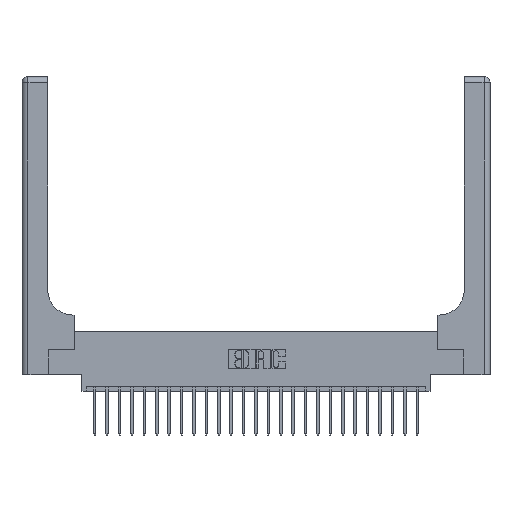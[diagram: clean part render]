
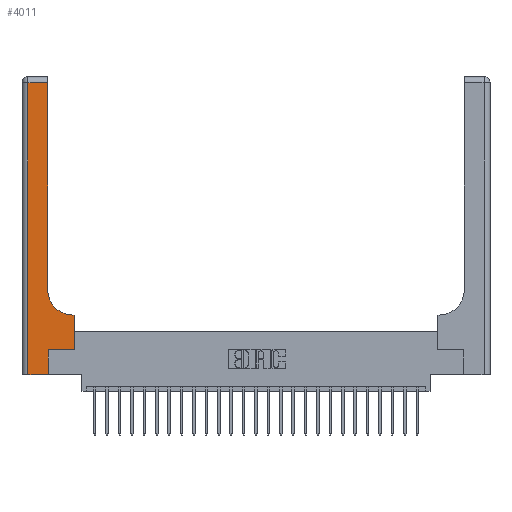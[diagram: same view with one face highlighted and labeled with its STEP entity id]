
A CAD part, top view. The second image highlights one B-rep face of the part: STEP entity #4011.
In plain terms, the highlighted planar face has unit normal (0, 0, 1).
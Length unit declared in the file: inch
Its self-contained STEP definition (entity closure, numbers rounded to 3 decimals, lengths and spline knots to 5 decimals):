
#607 = EDGE_CURVE ( 'NONE', #18740, #5531, #4757, .T. ) ;
#1061 = CARTESIAN_POINT ( 'NONE',  ( 0., 0., 0.37 ) ) ;
#1181 = DIRECTION ( 'NONE',  ( 0., 0., -1. ) ) ;
#1553 = VECTOR ( 'NONE', #13755, 39.37008 ) ;
#1917 = EDGE_CURVE ( 'NONE', #15763, #5478, #7448, .T. ) ;
#3031 = DIRECTION ( 'NONE',  ( 1., 0., 0. ) ) ;
#3609 = LINE ( 'NONE', #18284, #18433 ) ;
#4011 = ADVANCED_FACE ( 'NONE', ( #15959 ), #17779, .F. ) ;
#4052 = DIRECTION ( 'NONE',  ( -1., 0., 0. ) ) ;
#4178 = VERTEX_POINT ( 'NONE', #22391 ) ;
#4524 = EDGE_CURVE ( 'NONE', #15394, #18740, #11393, .T. ) ;
#4541 = CARTESIAN_POINT ( 'NONE',  ( 0.265, 0.25, 0.37 ) ) ;
#4726 = DIRECTION ( 'NONE',  ( 0., -1., 0. ) ) ;
#4745 = DIRECTION ( 'NONE',  ( 0., 1., 0. ) ) ;
#4757 = LINE ( 'NONE', #12441, #24632 ) ;
#4801 = LINE ( 'NONE', #1061, #14484 ) ;
#5115 = CARTESIAN_POINT ( 'NONE',  ( 0.26, 0.85, 0.37 ) ) ;
#5478 = VERTEX_POINT ( 'NONE', #5115 ) ;
#5531 = VERTEX_POINT ( 'NONE', #20825 ) ;
#5740 = VECTOR ( 'NONE', #16269, 39.37008 ) ;
#6201 = DIRECTION ( 'NONE',  ( 0., 0., -1. ) ) ;
#7081 = CARTESIAN_POINT ( 'NONE',  ( 0.528, 0.25, 0.37 ) ) ;
#7318 = LINE ( 'NONE', #11815, #1553 ) ;
#7344 = VERTEX_POINT ( 'NONE', #21788 ) ;
#7448 = CIRCLE ( 'NONE', #7459, 0.25 ) ;
#7459 = AXIS2_PLACEMENT_3D ( 'NONE', #12795, #1181, #14747 ) ;
#8339 = CARTESIAN_POINT ( 'NONE',  ( 0.26, 0.6, 0.37 ) ) ;
#9233 = EDGE_CURVE ( 'NONE', #22363, #7344, #16658, .T. ) ;
#9791 = CARTESIAN_POINT ( 'NONE',  ( 0.26, 2.94, 0.37 ) ) ;
#9891 = LINE ( 'NONE', #8339, #16274 ) ;
#9905 = EDGE_CURVE ( 'NONE', #4178, #22363, #22599, .T. ) ;
#10010 = CARTESIAN_POINT ( 'NONE',  ( 0., 3., 0.37 ) ) ;
#10056 = EDGE_CURVE ( 'NONE', #5531, #14721, #4801, .T. ) ;
#11393 = LINE ( 'NONE', #17607, #15332 ) ;
#11815 = CARTESIAN_POINT ( 'NONE',  ( 0.26, 3., 0.37 ) ) ;
#12441 = CARTESIAN_POINT ( 'NONE',  ( 0.06, 3., 0.37 ) ) ;
#12487 = EDGE_LOOP ( 'NONE', ( #17109, #17178, #18302, #18537, #19178, #19501, #20147, #20530, #21259 ) ) ;
#12795 = CARTESIAN_POINT ( 'NONE',  ( 0.51, 0.85, 0.37 ) ) ;
#12972 = VECTOR ( 'NONE', #18075, 39.37008 ) ;
#13468 = EDGE_CURVE ( 'NONE', #7344, #15763, #9891, .T. ) ;
#13755 = DIRECTION ( 'NONE',  ( 0., 1., 0. ) ) ;
#14301 = CARTESIAN_POINT ( 'NONE',  ( 0.528, 0.25, 0.37 ) ) ;
#14484 = VECTOR ( 'NONE', #3031, 39.37008 ) ;
#14721 = VERTEX_POINT ( 'NONE', #23700 ) ;
#14747 = DIRECTION ( 'NONE',  ( 1., 0., 0. ) ) ;
#15332 = VECTOR ( 'NONE', #4052, 39.37008 ) ;
#15394 = VERTEX_POINT ( 'NONE', #9791 ) ;
#15732 = CARTESIAN_POINT ( 'NONE',  ( 0.06, 2.94, 0.37 ) ) ;
#15763 = VERTEX_POINT ( 'NONE', #24397 ) ;
#15959 = FACE_OUTER_BOUND ( 'NONE', #12487, .T. ) ;
#16269 = DIRECTION ( 'NONE',  ( 0., 1., 0. ) ) ;
#16274 = VECTOR ( 'NONE', #21846, 39.37008 ) ;
#16658 = LINE ( 'NONE', #14301, #5740 ) ;
#17109 = ORIENTED_EDGE ( 'NONE', *, *, #22631, .T. ) ;
#17178 = ORIENTED_EDGE ( 'NONE', *, *, #4524, .T. ) ;
#17607 = CARTESIAN_POINT ( 'NONE',  ( 0., 2.94, 0.37 ) ) ;
#17779 = PLANE ( 'NONE',  #22672 ) ;
#18075 = DIRECTION ( 'NONE',  ( 1., 0., 0. ) ) ;
#18284 = CARTESIAN_POINT ( 'NONE',  ( 0.265, 0., 0.37 ) ) ;
#18302 = ORIENTED_EDGE ( 'NONE', *, *, #607, .T. ) ;
#18321 = EDGE_CURVE ( 'NONE', #14721, #4178, #3609, .T. ) ;
#18433 = VECTOR ( 'NONE', #4745, 39.37008 ) ;
#18537 = ORIENTED_EDGE ( 'NONE', *, *, #10056, .T. ) ;
#18740 = VERTEX_POINT ( 'NONE', #15732 ) ;
#19178 = ORIENTED_EDGE ( 'NONE', *, *, #18321, .T. ) ;
#19501 = ORIENTED_EDGE ( 'NONE', *, *, #9905, .T. ) ;
#19719 = DIRECTION ( 'NONE',  ( -1., 0., 0. ) ) ;
#20147 = ORIENTED_EDGE ( 'NONE', *, *, #9233, .T. ) ;
#20530 = ORIENTED_EDGE ( 'NONE', *, *, #13468, .T. ) ;
#20825 = CARTESIAN_POINT ( 'NONE',  ( 0.06, 0., 0.37 ) ) ;
#21259 = ORIENTED_EDGE ( 'NONE', *, *, #1917, .T. ) ;
#21788 = CARTESIAN_POINT ( 'NONE',  ( 0.528, 0.6, 0.37 ) ) ;
#21846 = DIRECTION ( 'NONE',  ( -1., 0., 0. ) ) ;
#22363 = VERTEX_POINT ( 'NONE', #7081 ) ;
#22391 = CARTESIAN_POINT ( 'NONE',  ( 0.265, 0.25, 0.37 ) ) ;
#22599 = LINE ( 'NONE', #4541, #12972 ) ;
#22631 = EDGE_CURVE ( 'NONE', #5478, #15394, #7318, .T. ) ;
#22672 = AXIS2_PLACEMENT_3D ( 'NONE', #10010, #6201, #19719 ) ;
#23700 = CARTESIAN_POINT ( 'NONE',  ( 0.265, 0., 0.37 ) ) ;
#24397 = CARTESIAN_POINT ( 'NONE',  ( 0.51, 0.6, 0.37 ) ) ;
#24632 = VECTOR ( 'NONE', #4726, 39.37008 ) ;
